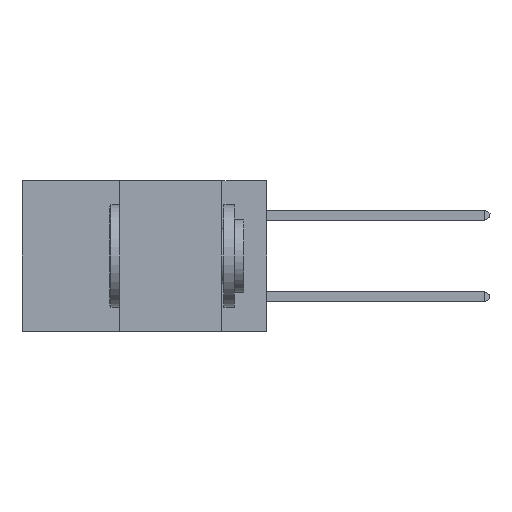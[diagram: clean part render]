
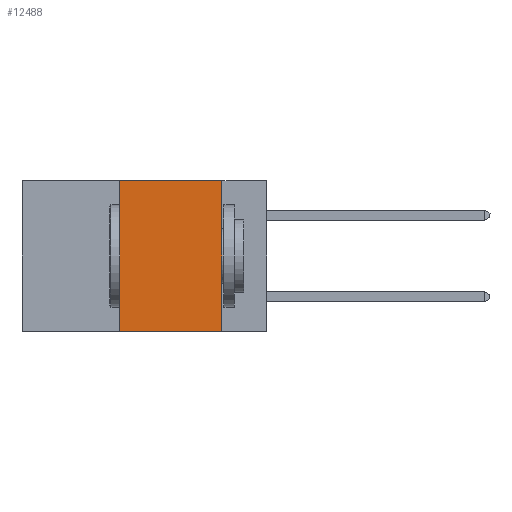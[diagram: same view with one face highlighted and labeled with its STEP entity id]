
A CAD part, left-side view. The second image highlights one B-rep face of the part: STEP entity #12488.
In plain terms, the highlighted planar face has unit normal (-1, 0, 0).
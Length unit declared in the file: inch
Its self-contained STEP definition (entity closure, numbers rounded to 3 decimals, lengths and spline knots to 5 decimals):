
#5 = CARTESIAN_POINT ( 'NONE',  ( 0., 0.11, -0.37 ) ) ;
#312 = EDGE_CURVE ( 'NONE', #9692, #897, #1347, .T. ) ;
#897 = VERTEX_POINT ( 'NONE', #14321 ) ;
#1155 = ORIENTED_EDGE ( 'NONE', *, *, #13135, .F. ) ;
#1347 = LINE ( 'NONE', #2604, #6997 ) ;
#1499 = FACE_OUTER_BOUND ( 'NONE', #9772, .T. ) ;
#1832 = CARTESIAN_POINT ( 'NONE',  ( 0., 0.11, 0. ) ) ;
#2604 = CARTESIAN_POINT ( 'NONE',  ( 0., 0.36, 0. ) ) ;
#2814 = DIRECTION ( 'NONE',  ( 0., -1., 0. ) ) ;
#2877 = CARTESIAN_POINT ( 'NONE',  ( 0., 0.6, 0. ) ) ;
#3530 = VECTOR ( 'NONE', #2814, 39.37008 ) ;
#4474 = LINE ( 'NONE', #11452, #7546 ) ;
#4476 = EDGE_CURVE ( 'NONE', #897, #7479, #6677, .T. ) ;
#4882 = VERTEX_POINT ( 'NONE', #5 ) ;
#5072 = DIRECTION ( 'NONE',  ( 0., 0., 1. ) ) ;
#5373 = PLANE ( 'NONE',  #12745 ) ;
#6494 = ORIENTED_EDGE ( 'NONE', *, *, #11121, .T. ) ;
#6501 = DIRECTION ( 'NONE',  ( 0., 0., -1. ) ) ;
#6587 = DIRECTION ( 'NONE',  ( 0., 0., -1. ) ) ;
#6677 = LINE ( 'NONE', #2877, #3530 ) ;
#6997 = VECTOR ( 'NONE', #5072, 39.37008 ) ;
#7479 = VERTEX_POINT ( 'NONE', #11606 ) ;
#7546 = VECTOR ( 'NONE', #9250, 39.37008 ) ;
#8412 = LINE ( 'NONE', #1832, #13825 ) ;
#8776 = CARTESIAN_POINT ( 'NONE',  ( 0., 0.6, 0. ) ) ;
#9250 = DIRECTION ( 'NONE',  ( 0., -1., 0. ) ) ;
#9692 = VERTEX_POINT ( 'NONE', #12253 ) ;
#9772 = EDGE_LOOP ( 'NONE', ( #1155, #9923, #10858, #6494 ) ) ;
#9923 = ORIENTED_EDGE ( 'NONE', *, *, #4476, .F. ) ;
#10858 = ORIENTED_EDGE ( 'NONE', *, *, #312, .F. ) ;
#11121 = EDGE_CURVE ( 'NONE', #9692, #4882, #4474, .T. ) ;
#11452 = CARTESIAN_POINT ( 'NONE',  ( 0., 0.6, -0.37 ) ) ;
#11606 = CARTESIAN_POINT ( 'NONE',  ( 0., 0.11, 0. ) ) ;
#12253 = CARTESIAN_POINT ( 'NONE',  ( 0., 0.36, -0.37 ) ) ;
#12488 = ADVANCED_FACE ( 'NONE', ( #1499 ), #5373, .F. ) ;
#12745 = AXIS2_PLACEMENT_3D ( 'NONE', #8776, #13133, #6501 ) ;
#13133 = DIRECTION ( 'NONE',  ( 1., 0., 0. ) ) ;
#13135 = EDGE_CURVE ( 'NONE', #7479, #4882, #8412, .T. ) ;
#13825 = VECTOR ( 'NONE', #6587, 39.37008 ) ;
#14321 = CARTESIAN_POINT ( 'NONE',  ( 0., 0.36, 0. ) ) ;
